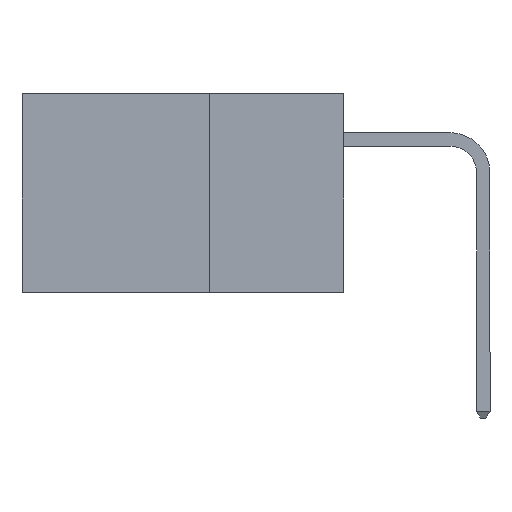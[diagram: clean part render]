
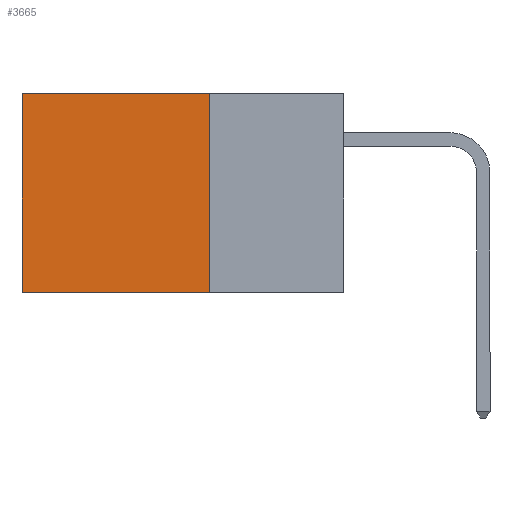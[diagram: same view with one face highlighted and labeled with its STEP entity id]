
A CAD part, left-side view. The second image highlights one B-rep face of the part: STEP entity #3665.
In plain terms, the highlighted planar face has unit normal (-1, 0, 0).
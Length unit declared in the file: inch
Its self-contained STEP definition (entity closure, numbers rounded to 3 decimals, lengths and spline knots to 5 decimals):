
#18 = EDGE_LOOP ( 'NONE', ( #8417, #4193, #8704, #5851 ) ) ;
#112 = LINE ( 'NONE', #2439, #5725 ) ;
#603 = VECTOR ( 'NONE', #4221, 39.37008 ) ;
#800 = VERTEX_POINT ( 'NONE', #2965 ) ;
#969 = LINE ( 'NONE', #7516, #8290 ) ;
#1545 = EDGE_CURVE ( 'NONE', #800, #2334, #6422, .T. ) ;
#1666 = VECTOR ( 'NONE', #2452, 39.37008 ) ;
#2334 = VERTEX_POINT ( 'NONE', #9211 ) ;
#2439 = CARTESIAN_POINT ( 'NONE',  ( 0.298, 0.25, 0. ) ) ;
#2452 = DIRECTION ( 'NONE',  ( 0., 0., -1. ) ) ;
#2965 = CARTESIAN_POINT ( 'NONE',  ( 0.298, 0.25, 0. ) ) ;
#3483 = FACE_OUTER_BOUND ( 'NONE', #18, .T. ) ;
#3665 = ADVANCED_FACE ( 'NONE', ( #3483 ), #8472, .F. ) ;
#3768 = CARTESIAN_POINT ( 'NONE',  ( 0.298, 0.6, 0. ) ) ;
#3931 = CARTESIAN_POINT ( 'NONE',  ( 0.298, 0.6, 0. ) ) ;
#3932 = EDGE_CURVE ( 'NONE', #2334, #4745, #969, .T. ) ;
#4193 = ORIENTED_EDGE ( 'NONE', *, *, #3932, .F. ) ;
#4221 = DIRECTION ( 'NONE',  ( 0., 0., -1. ) ) ;
#4344 = LINE ( 'NONE', #3931, #1666 ) ;
#4598 = DIRECTION ( 'NONE',  ( 0., 1., 0. ) ) ;
#4745 = VERTEX_POINT ( 'NONE', #7837 ) ;
#5725 = VECTOR ( 'NONE', #8761, 39.37008 ) ;
#5851 = ORIENTED_EDGE ( 'NONE', *, *, #6403, .T. ) ;
#6369 = CARTESIAN_POINT ( 'NONE',  ( 0.298, 0.25, 0. ) ) ;
#6403 = EDGE_CURVE ( 'NONE', #800, #8077, #112, .T. ) ;
#6422 = LINE ( 'NONE', #6369, #603 ) ;
#7144 = CARTESIAN_POINT ( 'NONE',  ( 0.298, 0.25, 0. ) ) ;
#7516 = CARTESIAN_POINT ( 'NONE',  ( 0.298, 0.25, -0.37 ) ) ;
#7837 = CARTESIAN_POINT ( 'NONE',  ( 0.298, 0.6, -0.37 ) ) ;
#8077 = VERTEX_POINT ( 'NONE', #3768 ) ;
#8229 = EDGE_CURVE ( 'NONE', #8077, #4745, #4344, .T. ) ;
#8290 = VECTOR ( 'NONE', #4598, 39.37008 ) ;
#8294 = AXIS2_PLACEMENT_3D ( 'NONE', #7144, #8909, #8738 ) ;
#8417 = ORIENTED_EDGE ( 'NONE', *, *, #8229, .T. ) ;
#8472 = PLANE ( 'NONE',  #8294 ) ;
#8704 = ORIENTED_EDGE ( 'NONE', *, *, #1545, .F. ) ;
#8738 = DIRECTION ( 'NONE',  ( 0., 0., -1. ) ) ;
#8761 = DIRECTION ( 'NONE',  ( 0., 1., 0. ) ) ;
#8909 = DIRECTION ( 'NONE',  ( 1., 0., 0. ) ) ;
#9211 = CARTESIAN_POINT ( 'NONE',  ( 0.298, 0.25, -0.37 ) ) ;
